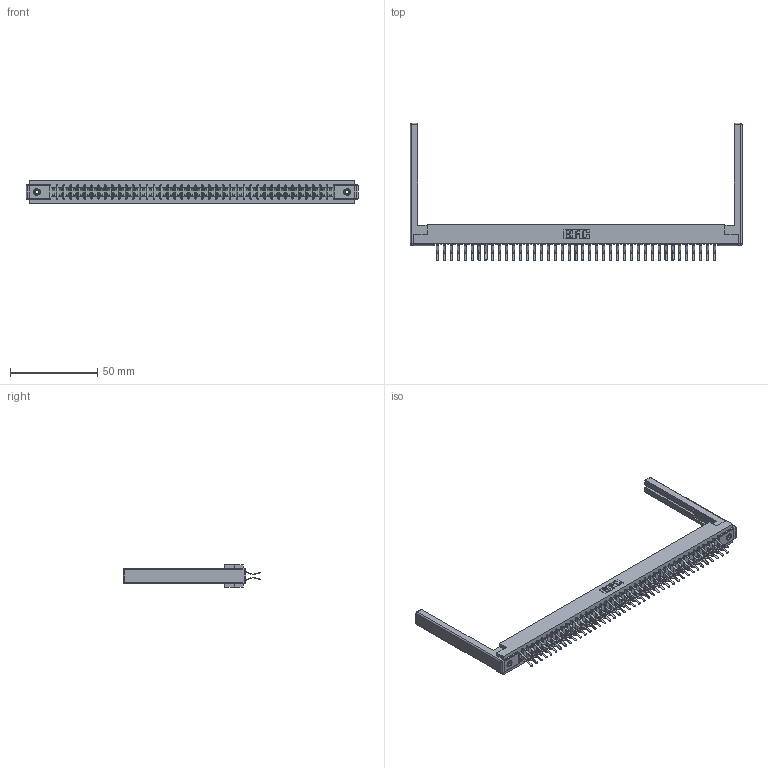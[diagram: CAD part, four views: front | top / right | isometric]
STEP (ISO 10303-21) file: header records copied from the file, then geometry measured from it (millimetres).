
FILE_DESCRIPTION (( 'STEP AP203' ), '1' );
FILE_NAME ('307-082-560-268.STEP', '2019-09-07T01:22:23', ( '' ), ( '' ), 'SwSTEP 2.0', 'SolidWorks 2016', '' );
FILE_SCHEMA (( 'CONFIG_CONTROL_DESIGN' ));
Length unit declared in the file: inch
Products named in the file (5): 307-220-068; 307-082-560-268; 307-290-001_560; 345-250-001_345-250-001-102; 307 Part_.156 Dia Mounting Holes
Assembly tree (87 placements, depth 2):
  307-082-560-268
    307 Part_.156 Dia Mounting Holes
    307-290-001_560  x82
    307-220-068  x2
    345-250-001_345-250-001-102  x2
Bounding box: 189.89 x 78.69 x 12.7 mm (x, y, z)
Volume: 24668.3 mm3; surface area: 29335.2 mm2
Topology: 87 solids, 87 shells, 4414 faces, 12357 edges, 7994 vertices
Faces by surface type: plane 2864, cylinder 1442, sphere 92, cone 12, torus 4
Entity records: 39447 total; most frequent: CARTESIAN_POINT 6430, ORIENTED_EDGE 6364, DIRECTION 6314, EDGE_CURVE 3182, VECTOR 2438, LINE 2438, VERTEX_POINT 2054, AXIS2_PLACEMENT_3D 1938
